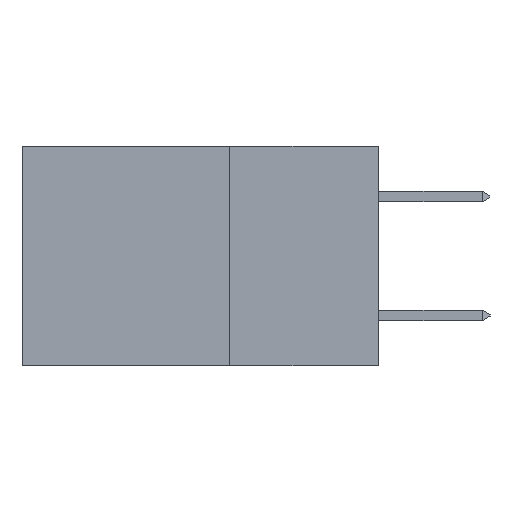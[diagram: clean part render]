
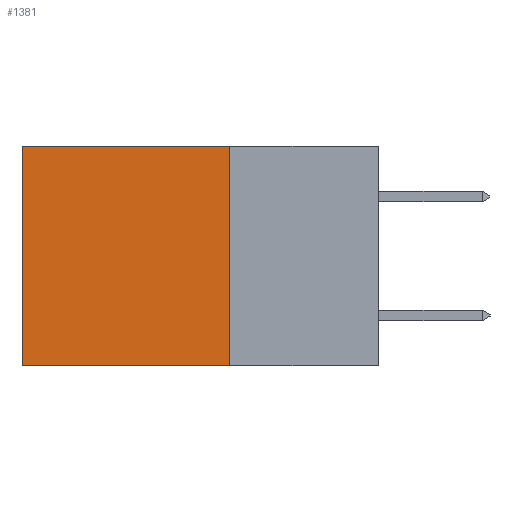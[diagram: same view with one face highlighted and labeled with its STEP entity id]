
A CAD part, left-side view. The second image highlights one B-rep face of the part: STEP entity #1381.
In plain terms, the highlighted planar face has unit normal (-1, 0, 0).
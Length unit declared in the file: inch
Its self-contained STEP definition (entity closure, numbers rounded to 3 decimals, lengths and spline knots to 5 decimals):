
#15 = VERTEX_POINT ( 'NONE', #6985 ) ;
#509 = PLANE ( 'NONE',  #1544 ) ;
#1381 = ADVANCED_FACE ( 'NONE', ( #11900 ), #509, .F. ) ;
#1406 = CARTESIAN_POINT ( 'NONE',  ( 0.2615, 0.25, -0.37 ) ) ;
#1544 = AXIS2_PLACEMENT_3D ( 'NONE', #1406, #6803, #7903 ) ;
#2494 = CARTESIAN_POINT ( 'NONE',  ( 0.2615, 0.25, -0.37 ) ) ;
#2507 = ORIENTED_EDGE ( 'NONE', *, *, #6302, .T. ) ;
#3797 = CARTESIAN_POINT ( 'NONE',  ( 0.2615, 0.25, 0. ) ) ;
#3832 = DIRECTION ( 'NONE',  ( 0., 0., -1. ) ) ;
#4054 = VECTOR ( 'NONE', #8425, 39.37008 ) ;
#4280 = EDGE_CURVE ( 'NONE', #5899, #15, #9071, .T. ) ;
#4338 = LINE ( 'NONE', #3797, #4054 ) ;
#4941 = VERTEX_POINT ( 'NONE', #9304 ) ;
#5319 = LINE ( 'NONE', #9397, #5615 ) ;
#5480 = CARTESIAN_POINT ( 'NONE',  ( 0.2615, 0.6, -0.37 ) ) ;
#5615 = VECTOR ( 'NONE', #3832, 39.37008 ) ;
#5899 = VERTEX_POINT ( 'NONE', #6051 ) ;
#6051 = CARTESIAN_POINT ( 'NONE',  ( 0.2615, 0.25, 0. ) ) ;
#6153 = VERTEX_POINT ( 'NONE', #5480 ) ;
#6302 = EDGE_CURVE ( 'NONE', #4941, #6153, #5319, .T. ) ;
#6333 = EDGE_LOOP ( 'NONE', ( #2507, #8636, #6593, #9794 ) ) ;
#6593 = ORIENTED_EDGE ( 'NONE', *, *, #4280, .F. ) ;
#6803 = DIRECTION ( 'NONE',  ( 1., 0., 0. ) ) ;
#6985 = CARTESIAN_POINT ( 'NONE',  ( 0.2615, 0.25, -0.37 ) ) ;
#7421 = LINE ( 'NONE', #2494, #11416 ) ;
#7903 = DIRECTION ( 'NONE',  ( 0., 0., -1. ) ) ;
#8135 = EDGE_CURVE ( 'NONE', #5899, #4941, #4338, .T. ) ;
#8425 = DIRECTION ( 'NONE',  ( 0., 1., 0. ) ) ;
#8636 = ORIENTED_EDGE ( 'NONE', *, *, #11020, .F. ) ;
#9071 = LINE ( 'NONE', #9196, #11221 ) ;
#9196 = CARTESIAN_POINT ( 'NONE',  ( 0.2615, 0.25, -0.37 ) ) ;
#9304 = CARTESIAN_POINT ( 'NONE',  ( 0.2615, 0.6, 0. ) ) ;
#9397 = CARTESIAN_POINT ( 'NONE',  ( 0.2615, 0.6, -0.37 ) ) ;
#9794 = ORIENTED_EDGE ( 'NONE', *, *, #8135, .T. ) ;
#9906 = DIRECTION ( 'NONE',  ( 0., 1., 0. ) ) ;
#10192 = DIRECTION ( 'NONE',  ( 0., 0., -1. ) ) ;
#11020 = EDGE_CURVE ( 'NONE', #15, #6153, #7421, .T. ) ;
#11221 = VECTOR ( 'NONE', #10192, 39.37008 ) ;
#11416 = VECTOR ( 'NONE', #9906, 39.37008 ) ;
#11900 = FACE_OUTER_BOUND ( 'NONE', #6333, .T. ) ;
